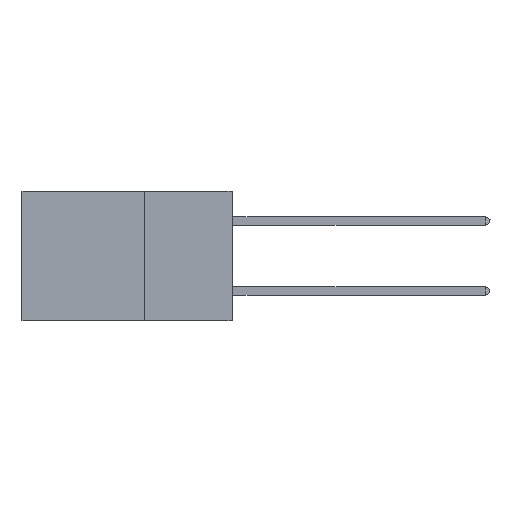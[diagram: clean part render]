
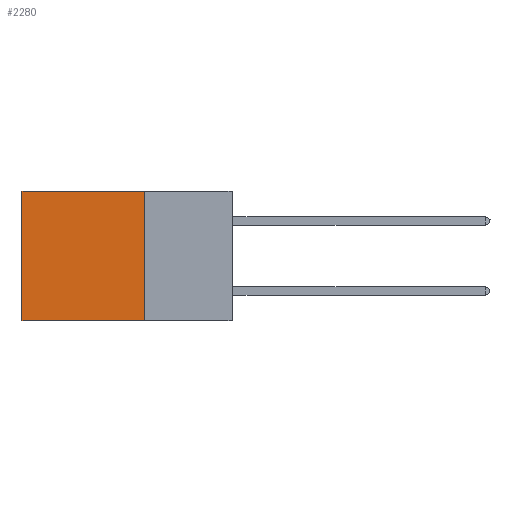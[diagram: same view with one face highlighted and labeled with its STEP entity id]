
A CAD part, left-side view. The second image highlights one B-rep face of the part: STEP entity #2280.
In plain terms, the highlighted planar face has unit normal (-1, 0, 0).
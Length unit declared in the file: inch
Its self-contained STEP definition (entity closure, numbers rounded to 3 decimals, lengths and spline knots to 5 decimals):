
#258 = LINE ( 'NONE', #2576, #26605 ) ;
#1799 = DIRECTION ( 'NONE',  ( 1., 0., 0. ) ) ;
#1850 = CARTESIAN_POINT ( 'NONE',  ( 0.2875, 0.6, 0. ) ) ;
#2092 = CARTESIAN_POINT ( 'NONE',  ( 0.2875, 0.6, -0.37 ) ) ;
#2280 = ADVANCED_FACE ( 'NONE', ( #5993 ), #17885, .F. ) ;
#2576 = CARTESIAN_POINT ( 'NONE',  ( 0.2875, 0.25, 0. ) ) ;
#3171 = DIRECTION ( 'NONE',  ( 0., 1., 0. ) ) ;
#5791 = ORIENTED_EDGE ( 'NONE', *, *, #13226, .T. ) ;
#5993 = FACE_OUTER_BOUND ( 'NONE', #6443, .T. ) ;
#6443 = EDGE_LOOP ( 'NONE', ( #6721, #17641, #16023, #5791 ) ) ;
#6721 = ORIENTED_EDGE ( 'NONE', *, *, #26424, .T. ) ;
#7272 = DIRECTION ( 'NONE',  ( 0., 1., 0. ) ) ;
#7346 = LINE ( 'NONE', #10862, #14151 ) ;
#9164 = CARTESIAN_POINT ( 'NONE',  ( 0.2875, 0.25, 0. ) ) ;
#9628 = EDGE_CURVE ( 'NONE', #22138, #26350, #7346, .T. ) ;
#10862 = CARTESIAN_POINT ( 'NONE',  ( 0.2875, 0.25, -0.37 ) ) ;
#11171 = AXIS2_PLACEMENT_3D ( 'NONE', #14375, #1799, #26417 ) ;
#12485 = VERTEX_POINT ( 'NONE', #13603 ) ;
#13226 = EDGE_CURVE ( 'NONE', #12485, #15122, #25544, .T. ) ;
#13603 = CARTESIAN_POINT ( 'NONE',  ( 0.2875, 0.25, 0. ) ) ;
#14151 = VECTOR ( 'NONE', #3171, 39.37008 ) ;
#14375 = CARTESIAN_POINT ( 'NONE',  ( 0.2875, 0.25, 0. ) ) ;
#15122 = VERTEX_POINT ( 'NONE', #1850 ) ;
#16023 = ORIENTED_EDGE ( 'NONE', *, *, #17891, .F. ) ;
#16127 = VECTOR ( 'NONE', #7272, 39.37008 ) ;
#17641 = ORIENTED_EDGE ( 'NONE', *, *, #9628, .F. ) ;
#17885 = PLANE ( 'NONE',  #11171 ) ;
#17891 = EDGE_CURVE ( 'NONE', #12485, #22138, #258, .T. ) ;
#21153 = DIRECTION ( 'NONE',  ( 0., 0., -1. ) ) ;
#22138 = VERTEX_POINT ( 'NONE', #26327 ) ;
#23298 = CARTESIAN_POINT ( 'NONE',  ( 0.2875, 0.6, 0. ) ) ;
#24096 = VECTOR ( 'NONE', #21153, 39.37008 ) ;
#25016 = DIRECTION ( 'NONE',  ( 0., 0., -1. ) ) ;
#25544 = LINE ( 'NONE', #9164, #16127 ) ;
#25614 = LINE ( 'NONE', #23298, #24096 ) ;
#26327 = CARTESIAN_POINT ( 'NONE',  ( 0.2875, 0.25, -0.37 ) ) ;
#26350 = VERTEX_POINT ( 'NONE', #2092 ) ;
#26417 = DIRECTION ( 'NONE',  ( 0., 0., -1. ) ) ;
#26424 = EDGE_CURVE ( 'NONE', #15122, #26350, #25614, .T. ) ;
#26605 = VECTOR ( 'NONE', #25016, 39.37008 ) ;
